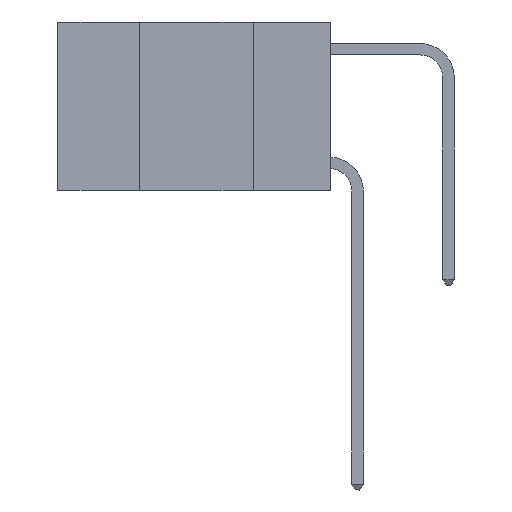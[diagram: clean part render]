
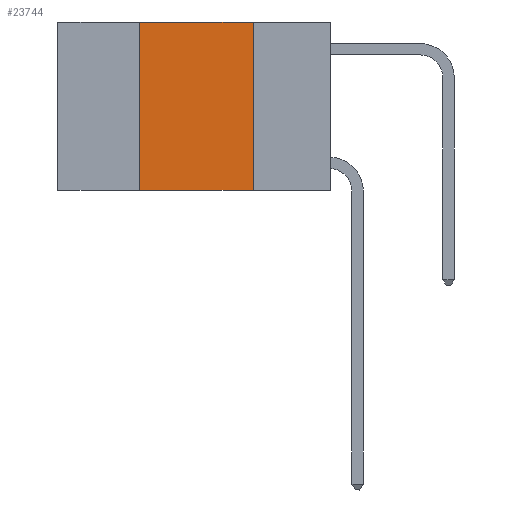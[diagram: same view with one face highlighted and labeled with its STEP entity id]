
A CAD part, left-side view. The second image highlights one B-rep face of the part: STEP entity #23744.
In plain terms, the highlighted planar face has unit normal (-1, 0, 0).
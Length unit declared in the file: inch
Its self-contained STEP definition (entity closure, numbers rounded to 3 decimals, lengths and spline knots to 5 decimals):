
#586 = CARTESIAN_POINT ( 'NONE',  ( 0., 0.17, 0. ) ) ;
#963 = LINE ( 'NONE', #9220, #32140 ) ;
#2504 = VECTOR ( 'NONE', #27899, 39.37008 ) ;
#4153 = EDGE_CURVE ( 'NONE', #28051, #8015, #25444, .T. ) ;
#6358 = EDGE_CURVE ( 'NONE', #8015, #32232, #963, .T. ) ;
#6454 = DIRECTION ( 'NONE',  ( 0., 0., 1. ) ) ;
#6568 = CARTESIAN_POINT ( 'NONE',  ( 0., 0.42, 0. ) ) ;
#6581 = CARTESIAN_POINT ( 'NONE',  ( 0., 0.17, 0. ) ) ;
#8015 = VERTEX_POINT ( 'NONE', #33486 ) ;
#8116 = CARTESIAN_POINT ( 'NONE',  ( 0., 0.6, 0. ) ) ;
#8349 = PLANE ( 'NONE',  #11461 ) ;
#8651 = EDGE_LOOP ( 'NONE', ( #17832, #21860, #23818, #10805 ) ) ;
#9220 = CARTESIAN_POINT ( 'NONE',  ( 0., 0.6, 0. ) ) ;
#10805 = ORIENTED_EDGE ( 'NONE', *, *, #31567, .T. ) ;
#10979 = LINE ( 'NONE', #25508, #2504 ) ;
#11461 = AXIS2_PLACEMENT_3D ( 'NONE', #8116, #23837, #29076 ) ;
#12200 = EDGE_CURVE ( 'NONE', #32232, #19042, #14063, .T. ) ;
#14063 = LINE ( 'NONE', #6581, #23344 ) ;
#15999 = FACE_OUTER_BOUND ( 'NONE', #8651, .T. ) ;
#16404 = DIRECTION ( 'NONE',  ( 0., 0., -1. ) ) ;
#17832 = ORIENTED_EDGE ( 'NONE', *, *, #12200, .F. ) ;
#18554 = VECTOR ( 'NONE', #6454, 39.37008 ) ;
#19042 = VERTEX_POINT ( 'NONE', #26782 ) ;
#19313 = CARTESIAN_POINT ( 'NONE',  ( 0., 0.42, -0.37 ) ) ;
#21860 = ORIENTED_EDGE ( 'NONE', *, *, #6358, .F. ) ;
#23344 = VECTOR ( 'NONE', #16404, 39.37008 ) ;
#23744 = ADVANCED_FACE ( 'NONE', ( #15999 ), #8349, .F. ) ;
#23818 = ORIENTED_EDGE ( 'NONE', *, *, #4153, .F. ) ;
#23837 = DIRECTION ( 'NONE',  ( 1., 0., 0. ) ) ;
#25444 = LINE ( 'NONE', #6568, #18554 ) ;
#25508 = CARTESIAN_POINT ( 'NONE',  ( 0., 0.6, -0.37 ) ) ;
#26782 = CARTESIAN_POINT ( 'NONE',  ( 0., 0.17, -0.37 ) ) ;
#27899 = DIRECTION ( 'NONE',  ( 0., -1., 0. ) ) ;
#28051 = VERTEX_POINT ( 'NONE', #19313 ) ;
#29076 = DIRECTION ( 'NONE',  ( 0., 0., -1. ) ) ;
#29132 = DIRECTION ( 'NONE',  ( 0., -1., 0. ) ) ;
#31567 = EDGE_CURVE ( 'NONE', #28051, #19042, #10979, .T. ) ;
#32140 = VECTOR ( 'NONE', #29132, 39.37008 ) ;
#32232 = VERTEX_POINT ( 'NONE', #586 ) ;
#33486 = CARTESIAN_POINT ( 'NONE',  ( 0., 0.42, 0. ) ) ;
